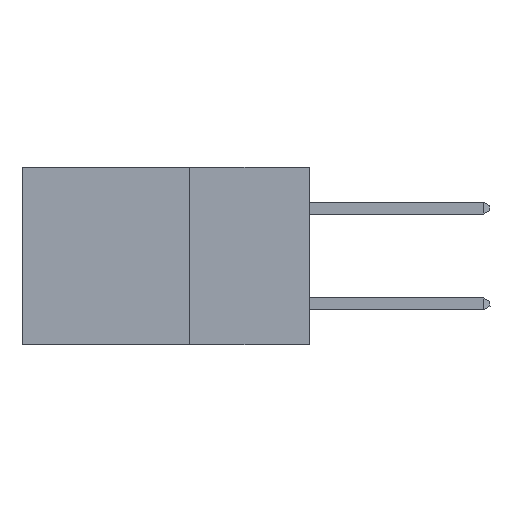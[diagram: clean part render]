
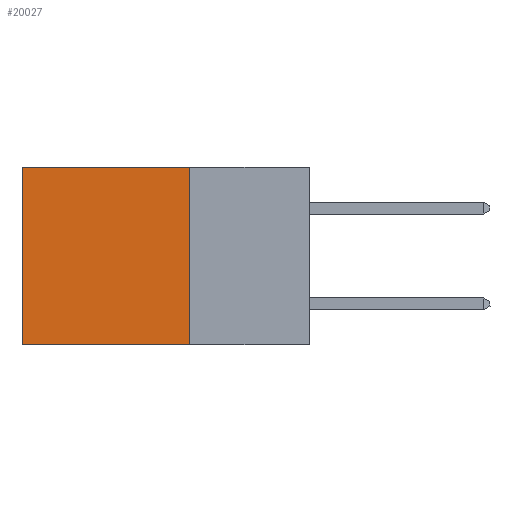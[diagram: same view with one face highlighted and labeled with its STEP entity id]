
A CAD part, left-side view. The second image highlights one B-rep face of the part: STEP entity #20027.
In plain terms, the highlighted planar face has unit normal (-1, 0, 0).
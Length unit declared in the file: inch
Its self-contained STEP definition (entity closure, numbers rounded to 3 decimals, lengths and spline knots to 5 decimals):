
#91 = CARTESIAN_POINT ( 'NONE',  ( 0.2875, 0.25, 0. ) ) ;
#718 = VERTEX_POINT ( 'NONE', #91 ) ;
#1159 = EDGE_CURVE ( 'NONE', #718, #9816, #3400, .T. ) ;
#1298 = PLANE ( 'NONE',  #8068 ) ;
#1767 = ORIENTED_EDGE ( 'NONE', *, *, #1159, .F. ) ;
#2392 = VECTOR ( 'NONE', #3462, 39.37008 ) ;
#2572 = ORIENTED_EDGE ( 'NONE', *, *, #7926, .F. ) ;
#3400 = LINE ( 'NONE', #14383, #19408 ) ;
#3462 = DIRECTION ( 'NONE',  ( 0., 1., 0. ) ) ;
#4556 = CARTESIAN_POINT ( 'NONE',  ( 0.2875, 0.25, 0. ) ) ;
#4732 = LINE ( 'NONE', #12940, #9025 ) ;
#4911 = VECTOR ( 'NONE', #12533, 39.37008 ) ;
#6108 = CARTESIAN_POINT ( 'NONE',  ( 0.2875, 0.25, 0. ) ) ;
#7795 = DIRECTION ( 'NONE',  ( 1., 0., 0. ) ) ;
#7926 = EDGE_CURVE ( 'NONE', #9816, #15589, #19444, .T. ) ;
#8068 = AXIS2_PLACEMENT_3D ( 'NONE', #4556, #7795, #18951 ) ;
#8688 = EDGE_LOOP ( 'NONE', ( #8774, #2572, #1767, #20246 ) ) ;
#8774 = ORIENTED_EDGE ( 'NONE', *, *, #18184, .T. ) ;
#9025 = VECTOR ( 'NONE', #14512, 39.37008 ) ;
#9146 = EDGE_CURVE ( 'NONE', #718, #16144, #9214, .T. ) ;
#9214 = LINE ( 'NONE', #6108, #4911 ) ;
#9816 = VERTEX_POINT ( 'NONE', #15628 ) ;
#12533 = DIRECTION ( 'NONE',  ( 0., 1., 0. ) ) ;
#12940 = CARTESIAN_POINT ( 'NONE',  ( 0.2875, 0.6, 0. ) ) ;
#14218 = DIRECTION ( 'NONE',  ( 0., 0., -1. ) ) ;
#14383 = CARTESIAN_POINT ( 'NONE',  ( 0.2875, 0.25, 0. ) ) ;
#14512 = DIRECTION ( 'NONE',  ( 0., 0., -1. ) ) ;
#14657 = CARTESIAN_POINT ( 'NONE',  ( 0.2875, 0.6, -0.37 ) ) ;
#15589 = VERTEX_POINT ( 'NONE', #14657 ) ;
#15628 = CARTESIAN_POINT ( 'NONE',  ( 0.2875, 0.25, -0.37 ) ) ;
#16144 = VERTEX_POINT ( 'NONE', #19191 ) ;
#16273 = CARTESIAN_POINT ( 'NONE',  ( 0.2875, 0.25, -0.37 ) ) ;
#18184 = EDGE_CURVE ( 'NONE', #16144, #15589, #4732, .T. ) ;
#18951 = DIRECTION ( 'NONE',  ( 0., 0., -1. ) ) ;
#19191 = CARTESIAN_POINT ( 'NONE',  ( 0.2875, 0.6, 0. ) ) ;
#19408 = VECTOR ( 'NONE', #14218, 39.37008 ) ;
#19444 = LINE ( 'NONE', #16273, #2392 ) ;
#19877 = FACE_OUTER_BOUND ( 'NONE', #8688, .T. ) ;
#20027 = ADVANCED_FACE ( 'NONE', ( #19877 ), #1298, .F. ) ;
#20246 = ORIENTED_EDGE ( 'NONE', *, *, #9146, .T. ) ;
